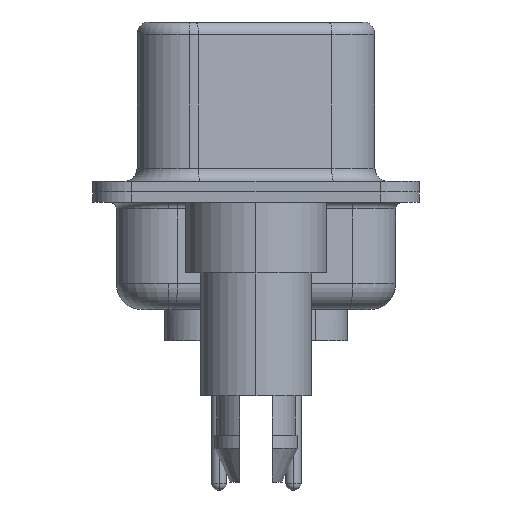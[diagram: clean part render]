
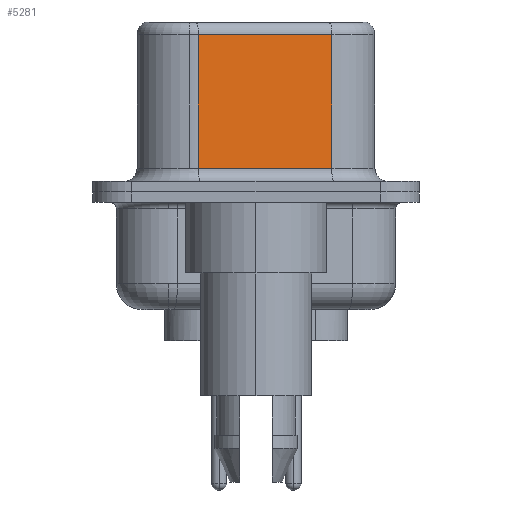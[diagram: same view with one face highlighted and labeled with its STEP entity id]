
A CAD part, left-side view. The second image highlights one B-rep face of the part: STEP entity #5281.
In plain terms, the highlighted planar face has unit normal (-0.985, -0.174, 0).
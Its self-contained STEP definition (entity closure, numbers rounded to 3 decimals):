
#158 = DIRECTION ( 'NONE',  ( 0., 0., -1. ) ) ;
#1078 = CARTESIAN_POINT ( 'NONE',  ( 4.58, -2.897, 0.9 ) ) ;
#2155 = VECTOR ( 'NONE', #3526, 1000. ) ;
#2457 = VERTEX_POINT ( 'NONE', #1078 ) ;
#2525 = VECTOR ( 'NONE', #14133, 1000. ) ;
#3083 = DIRECTION ( 'NONE',  ( 0., 0., -1. ) ) ;
#3526 = DIRECTION ( 'NONE',  ( -0.174, 0.985, 0. ) ) ;
#5281 = ADVANCED_FACE ( 'NONE', ( #15706 ), #18778, .F. ) ;
#5330 = CARTESIAN_POINT ( 'NONE',  ( 4.58, -2.897, 6.52 ) ) ;
#5715 = LINE ( 'NONE', #9229, #2525 ) ;
#5756 = EDGE_CURVE ( 'NONE', #16161, #2457, #6588, .T. ) ;
#6588 = LINE ( 'NONE', #6708, #17178 ) ;
#6708 = CARTESIAN_POINT ( 'NONE',  ( 4.58, -2.897, 6.52 ) ) ;
#7456 = VERTEX_POINT ( 'NONE', #18604 ) ;
#8037 = VECTOR ( 'NONE', #158, 1000. ) ;
#8297 = ORIENTED_EDGE ( 'NONE', *, *, #5756, .F. ) ;
#8462 = CARTESIAN_POINT ( 'NONE',  ( 4.58, -2.897, 6.02 ) ) ;
#9229 = CARTESIAN_POINT ( 'NONE',  ( 4.58, -2.897, 0.9 ) ) ;
#9909 = ORIENTED_EDGE ( 'NONE', *, *, #10629, .T. ) ;
#10158 = ORIENTED_EDGE ( 'NONE', *, *, #19001, .T. ) ;
#10595 = EDGE_CURVE ( 'NONE', #16161, #7456, #16759, .T. ) ;
#10629 = EDGE_CURVE ( 'NONE', #19781, #2457, #5715, .T. ) ;
#12230 = ORIENTED_EDGE ( 'NONE', *, *, #10595, .T. ) ;
#13381 = LINE ( 'NONE', #16892, #8037 ) ;
#14080 = DIRECTION ( 'NONE',  ( -0.174, 0.985, 0. ) ) ;
#14133 = DIRECTION ( 'NONE',  ( 0.174, -0.985, 0. ) ) ;
#15137 = CARTESIAN_POINT ( 'NONE',  ( 3.68, 2.203, 0.9 ) ) ;
#15415 = CARTESIAN_POINT ( 'NONE',  ( 4.58, -2.897, 6.02 ) ) ;
#15597 = DIRECTION ( 'NONE',  ( 0.985, 0.174, 0. ) ) ;
#15706 = FACE_OUTER_BOUND ( 'NONE', #17108, .T. ) ;
#16161 = VERTEX_POINT ( 'NONE', #15415 ) ;
#16759 = LINE ( 'NONE', #8462, #2155 ) ;
#16892 = CARTESIAN_POINT ( 'NONE',  ( 3.68, 2.203, 6.52 ) ) ;
#17108 = EDGE_LOOP ( 'NONE', ( #8297, #12230, #10158, #9909 ) ) ;
#17178 = VECTOR ( 'NONE', #3083, 1000. ) ;
#18604 = CARTESIAN_POINT ( 'NONE',  ( 3.68, 2.203, 6.02 ) ) ;
#18778 = PLANE ( 'NONE',  #21018 ) ;
#19001 = EDGE_CURVE ( 'NONE', #7456, #19781, #13381, .T. ) ;
#19781 = VERTEX_POINT ( 'NONE', #15137 ) ;
#21018 = AXIS2_PLACEMENT_3D ( 'NONE', #5330, #15597, #14080 ) ;
